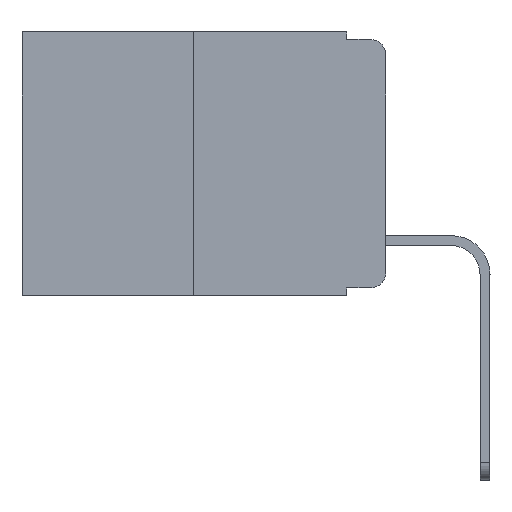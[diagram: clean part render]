
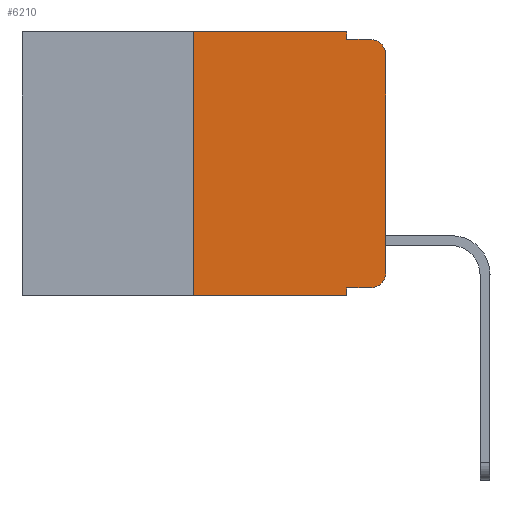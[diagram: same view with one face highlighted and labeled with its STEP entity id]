
A CAD part, left-side view. The second image highlights one B-rep face of the part: STEP entity #6210.
In plain terms, the highlighted planar face has unit normal (-1, 0, 0).
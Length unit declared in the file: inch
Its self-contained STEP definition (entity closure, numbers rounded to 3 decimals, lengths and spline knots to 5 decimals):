
#425 = AXIS2_PLACEMENT_3D ( 'NONE', #7242, #5791, #18355 ) ;
#1063 = DIRECTION ( 'NONE',  ( 0., 0., 1. ) ) ;
#1283 = CARTESIAN_POINT ( 'NONE',  ( 0., 0.473, -0.343 ) ) ;
#1585 = ORIENTED_EDGE ( 'NONE', *, *, #9916, .T. ) ;
#1705 = CARTESIAN_POINT ( 'NONE',  ( 0., 0.25, 0. ) ) ;
#1893 = CARTESIAN_POINT ( 'NONE',  ( 0., 0.051, -0.01 ) ) ;
#1981 = VERTEX_POINT ( 'NONE', #5888 ) ;
#2919 = EDGE_LOOP ( 'NONE', ( #14041, #18924, #8348, #9845, #9391, #16279, #12154, #13647, #8217, #1585 ) ) ;
#3283 = DIRECTION ( 'NONE',  ( 1., 0., 0. ) ) ;
#3316 = CIRCLE ( 'NONE', #425, 0.02 ) ;
#3886 = VERTEX_POINT ( 'NONE', #9656 ) ;
#3961 = LINE ( 'NONE', #17947, #13042 ) ;
#4039 = FACE_OUTER_BOUND ( 'NONE', #2919, .T. ) ;
#4265 = VERTEX_POINT ( 'NONE', #19554 ) ;
#4557 = LINE ( 'NONE', #8266, #17866 ) ;
#4712 = DIRECTION ( 'NONE',  ( 0., -1., 0. ) ) ;
#4981 = DIRECTION ( 'NONE',  ( 0., 0., 1. ) ) ;
#5791 = DIRECTION ( 'NONE',  ( -1., 0., 0. ) ) ;
#5815 = EDGE_CURVE ( 'NONE', #19424, #10750, #3316, .T. ) ;
#5888 = CARTESIAN_POINT ( 'NONE',  ( 0., 0.051, 0. ) ) ;
#6210 = ADVANCED_FACE ( 'NONE', ( #4039 ), #14122, .F. ) ;
#6318 = CARTESIAN_POINT ( 'NONE',  ( 0., 0.051, 0. ) ) ;
#6597 = DIRECTION ( 'NONE',  ( 0., 0., -1. ) ) ;
#6882 = VERTEX_POINT ( 'NONE', #17562 ) ;
#6917 = AXIS2_PLACEMENT_3D ( 'NONE', #17572, #14384, #6597 ) ;
#7185 = DIRECTION ( 'NONE',  ( 0., 0., -1. ) ) ;
#7242 = CARTESIAN_POINT ( 'NONE',  ( 0., 0.02, -0.03 ) ) ;
#7463 = VERTEX_POINT ( 'NONE', #1705 ) ;
#8217 = ORIENTED_EDGE ( 'NONE', *, *, #15516, .T. ) ;
#8266 = CARTESIAN_POINT ( 'NONE',  ( 0., 0., 0. ) ) ;
#8282 = DIRECTION ( 'NONE',  ( 0., -1., 0. ) ) ;
#8348 = ORIENTED_EDGE ( 'NONE', *, *, #16094, .F. ) ;
#8970 = EDGE_CURVE ( 'NONE', #12711, #3886, #13035, .T. ) ;
#9331 = VECTOR ( 'NONE', #7185, 39.37008 ) ;
#9391 = ORIENTED_EDGE ( 'NONE', *, *, #10301, .F. ) ;
#9656 = CARTESIAN_POINT ( 'NONE',  ( 0., 0.051, -0.343 ) ) ;
#9845 = ORIENTED_EDGE ( 'NONE', *, *, #19038, .F. ) ;
#9916 = EDGE_CURVE ( 'NONE', #18532, #4265, #13015, .T. ) ;
#10017 = CARTESIAN_POINT ( 'NONE',  ( 0., 0.02, -0.333 ) ) ;
#10095 = VECTOR ( 'NONE', #19115, 39.37008 ) ;
#10261 = CARTESIAN_POINT ( 'NONE',  ( 0., 0.051, -0.333 ) ) ;
#10301 = EDGE_CURVE ( 'NONE', #7463, #1981, #19429, .T. ) ;
#10654 = VECTOR ( 'NONE', #4712, 39.37008 ) ;
#10747 = CARTESIAN_POINT ( 'NONE',  ( 0., 0., -0.03 ) ) ;
#10750 = VERTEX_POINT ( 'NONE', #14692 ) ;
#11383 = CARTESIAN_POINT ( 'NONE',  ( 0., 0.25, 0. ) ) ;
#12028 = CARTESIAN_POINT ( 'NONE',  ( 0., 0.051, 0. ) ) ;
#12089 = EDGE_CURVE ( 'NONE', #4265, #19424, #4557, .T. ) ;
#12154 = ORIENTED_EDGE ( 'NONE', *, *, #13540, .T. ) ;
#12332 = VERTEX_POINT ( 'NONE', #17153 ) ;
#12535 = DIRECTION ( 'NONE',  ( 0., 0., -1. ) ) ;
#12677 = CARTESIAN_POINT ( 'NONE',  ( 0., 0.473, 0. ) ) ;
#12711 = VERTEX_POINT ( 'NONE', #10261 ) ;
#13015 = CIRCLE ( 'NONE', #6917, 0.02 ) ;
#13035 = LINE ( 'NONE', #12028, #9331 ) ;
#13042 = VECTOR ( 'NONE', #8282, 39.37008 ) ;
#13540 = EDGE_CURVE ( 'NONE', #12332, #3886, #17551, .T. ) ;
#13647 = ORIENTED_EDGE ( 'NONE', *, *, #8970, .F. ) ;
#14041 = ORIENTED_EDGE ( 'NONE', *, *, #12089, .T. ) ;
#14122 = PLANE ( 'NONE',  #20208 ) ;
#14255 = DIRECTION ( 'NONE',  ( 0., 0., -1. ) ) ;
#14265 = EDGE_CURVE ( 'NONE', #12332, #7463, #18759, .T. ) ;
#14384 = DIRECTION ( 'NONE',  ( -1., 0., 0. ) ) ;
#14548 = VECTOR ( 'NONE', #4981, 39.37008 ) ;
#14631 = VECTOR ( 'NONE', #12535, 39.37008 ) ;
#14692 = CARTESIAN_POINT ( 'NONE',  ( 0., 0.02, -0.01 ) ) ;
#15005 = LINE ( 'NONE', #1893, #10095 ) ;
#15260 = CARTESIAN_POINT ( 'NONE',  ( 0., 0.473, 0. ) ) ;
#15516 = EDGE_CURVE ( 'NONE', #12711, #18532, #3961, .T. ) ;
#16094 = EDGE_CURVE ( 'NONE', #6882, #10750, #15005, .T. ) ;
#16209 = VECTOR ( 'NONE', #18530, 39.37008 ) ;
#16279 = ORIENTED_EDGE ( 'NONE', *, *, #14265, .F. ) ;
#17153 = CARTESIAN_POINT ( 'NONE',  ( 0., 0.25, -0.343 ) ) ;
#17551 = LINE ( 'NONE', #1283, #10654 ) ;
#17562 = CARTESIAN_POINT ( 'NONE',  ( 0., 0.051, -0.01 ) ) ;
#17572 = CARTESIAN_POINT ( 'NONE',  ( 0., 0.02, -0.313 ) ) ;
#17851 = LINE ( 'NONE', #6318, #14631 ) ;
#17866 = VECTOR ( 'NONE', #1063, 39.37008 ) ;
#17947 = CARTESIAN_POINT ( 'NONE',  ( 0., 0.051, -0.333 ) ) ;
#18355 = DIRECTION ( 'NONE',  ( 0., 0., -1. ) ) ;
#18530 = DIRECTION ( 'NONE',  ( 0., -1., 0. ) ) ;
#18532 = VERTEX_POINT ( 'NONE', #10017 ) ;
#18759 = LINE ( 'NONE', #11383, #14548 ) ;
#18924 = ORIENTED_EDGE ( 'NONE', *, *, #5815, .T. ) ;
#19038 = EDGE_CURVE ( 'NONE', #1981, #6882, #17851, .T. ) ;
#19115 = DIRECTION ( 'NONE',  ( 0., -1., 0. ) ) ;
#19424 = VERTEX_POINT ( 'NONE', #10747 ) ;
#19429 = LINE ( 'NONE', #15260, #16209 ) ;
#19554 = CARTESIAN_POINT ( 'NONE',  ( 0., 0., -0.313 ) ) ;
#20208 = AXIS2_PLACEMENT_3D ( 'NONE', #12677, #3283, #14255 ) ;
